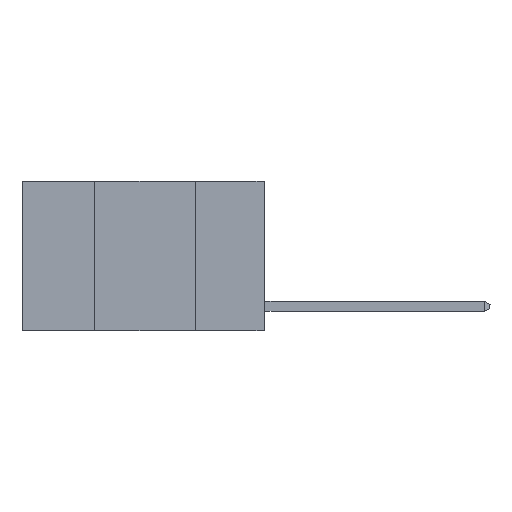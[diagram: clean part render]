
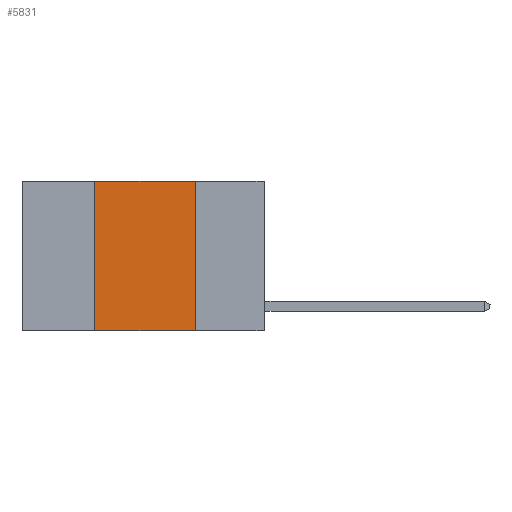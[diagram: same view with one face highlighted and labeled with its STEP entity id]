
A CAD part, left-side view. The second image highlights one B-rep face of the part: STEP entity #5831.
In plain terms, the highlighted planar face has unit normal (-1, 0, 0).
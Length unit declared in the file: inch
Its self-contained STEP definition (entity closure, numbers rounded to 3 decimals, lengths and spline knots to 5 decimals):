
#459 = PLANE ( 'NONE',  #13846 ) ;
#551 = EDGE_CURVE ( 'NONE', #11106, #12485, #8386, .T. ) ;
#582 = CARTESIAN_POINT ( 'NONE',  ( 0., 0.42, 0. ) ) ;
#1404 = CARTESIAN_POINT ( 'NONE',  ( 0., 0.6, 0. ) ) ;
#1417 = ORIENTED_EDGE ( 'NONE', *, *, #5691, .F. ) ;
#2502 = VERTEX_POINT ( 'NONE', #9951 ) ;
#2561 = CARTESIAN_POINT ( 'NONE',  ( 0., 0.17, -0.37 ) ) ;
#2625 = EDGE_LOOP ( 'NONE', ( #2947, #1417, #6513, #14830 ) ) ;
#2662 = CARTESIAN_POINT ( 'NONE',  ( 0., 0.42, 0. ) ) ;
#2947 = ORIENTED_EDGE ( 'NONE', *, *, #6441, .F. ) ;
#5363 = LINE ( 'NONE', #2662, #11986 ) ;
#5691 = EDGE_CURVE ( 'NONE', #14538, #2502, #14407, .T. ) ;
#5831 = ADVANCED_FACE ( 'NONE', ( #6955 ), #459, .F. ) ;
#6030 = DIRECTION ( 'NONE',  ( 0., -1., 0. ) ) ;
#6441 = EDGE_CURVE ( 'NONE', #2502, #12485, #6556, .T. ) ;
#6513 = ORIENTED_EDGE ( 'NONE', *, *, #11666, .F. ) ;
#6556 = LINE ( 'NONE', #11114, #14897 ) ;
#6955 = FACE_OUTER_BOUND ( 'NONE', #2625, .T. ) ;
#7140 = VECTOR ( 'NONE', #6030, 39.37008 ) ;
#7273 = VECTOR ( 'NONE', #14259, 39.37008 ) ;
#8386 = LINE ( 'NONE', #11971, #7273 ) ;
#8589 = DIRECTION ( 'NONE',  ( 0., 0., 1. ) ) ;
#8655 = DIRECTION ( 'NONE',  ( 0., 0., -1. ) ) ;
#9198 = CARTESIAN_POINT ( 'NONE',  ( 0., 0.42, -0.37 ) ) ;
#9951 = CARTESIAN_POINT ( 'NONE',  ( 0., 0.17, 0. ) ) ;
#11106 = VERTEX_POINT ( 'NONE', #9198 ) ;
#11114 = CARTESIAN_POINT ( 'NONE',  ( 0., 0.17, 0. ) ) ;
#11666 = EDGE_CURVE ( 'NONE', #11106, #14538, #5363, .T. ) ;
#11971 = CARTESIAN_POINT ( 'NONE',  ( 0., 0.6, -0.37 ) ) ;
#11986 = VECTOR ( 'NONE', #8589, 39.37008 ) ;
#12172 = DIRECTION ( 'NONE',  ( 1., 0., 0. ) ) ;
#12485 = VERTEX_POINT ( 'NONE', #2561 ) ;
#13366 = DIRECTION ( 'NONE',  ( 0., 0., -1. ) ) ;
#13428 = CARTESIAN_POINT ( 'NONE',  ( 0., 0.6, 0. ) ) ;
#13846 = AXIS2_PLACEMENT_3D ( 'NONE', #13428, #12172, #8655 ) ;
#14259 = DIRECTION ( 'NONE',  ( 0., -1., 0. ) ) ;
#14407 = LINE ( 'NONE', #1404, #7140 ) ;
#14538 = VERTEX_POINT ( 'NONE', #582 ) ;
#14830 = ORIENTED_EDGE ( 'NONE', *, *, #551, .T. ) ;
#14897 = VECTOR ( 'NONE', #13366, 39.37008 ) ;
